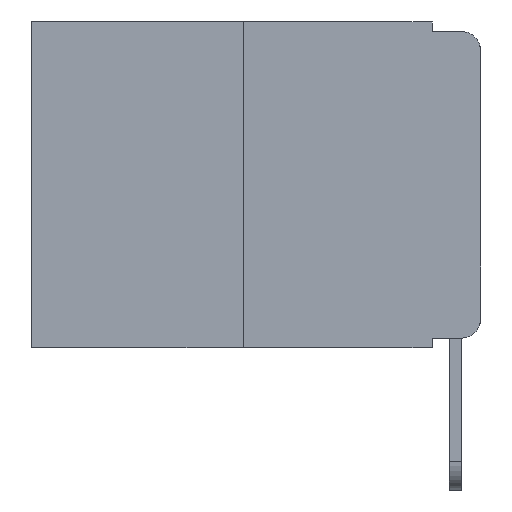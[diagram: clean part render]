
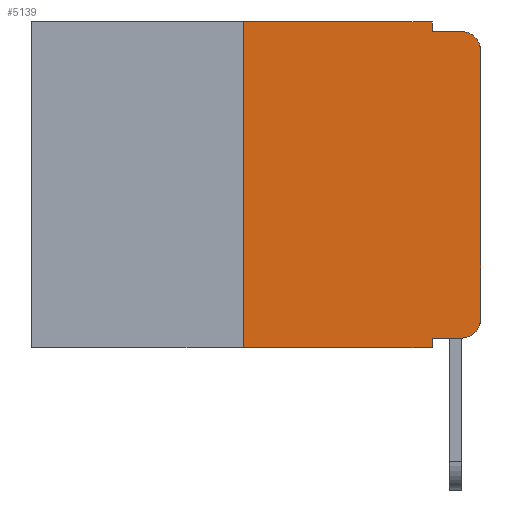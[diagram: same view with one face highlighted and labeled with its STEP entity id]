
A CAD part, left-side view. The second image highlights one B-rep face of the part: STEP entity #5139.
In plain terms, the highlighted planar face has unit normal (-1, 0, 0).
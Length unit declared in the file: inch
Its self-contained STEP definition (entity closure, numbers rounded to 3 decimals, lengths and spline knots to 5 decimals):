
#369 = DIRECTION ( 'NONE',  ( 0., 0., 1. ) ) ;
#731 = DIRECTION ( 'NONE',  ( 0., 0., 1. ) ) ;
#906 = AXIS2_PLACEMENT_3D ( 'NONE', #6692, #8714, #2921 ) ;
#1438 = VERTEX_POINT ( 'NONE', #13425 ) ;
#1613 = ORIENTED_EDGE ( 'NONE', *, *, #2578, .F. ) ;
#1664 = VERTEX_POINT ( 'NONE', #3669 ) ;
#1966 = CARTESIAN_POINT ( 'NONE',  ( 0., 0.051, 0. ) ) ;
#2036 = DIRECTION ( 'NONE',  ( 0., 0., -1. ) ) ;
#2057 = VERTEX_POINT ( 'NONE', #5916 ) ;
#2065 = EDGE_CURVE ( 'NONE', #4809, #1664, #3626, .T. ) ;
#2370 = EDGE_CURVE ( 'NONE', #10915, #11073, #7590, .T. ) ;
#2481 = CARTESIAN_POINT ( 'NONE',  ( 0., 0., -0.313 ) ) ;
#2497 = DIRECTION ( 'NONE',  ( 0., 0., -1. ) ) ;
#2549 = EDGE_CURVE ( 'NONE', #7358, #14684, #6705, .T. ) ;
#2551 = EDGE_CURVE ( 'NONE', #14684, #2057, #7060, .T. ) ;
#2554 = EDGE_CURVE ( 'NONE', #13820, #2057, #12006, .T. ) ;
#2575 = EDGE_CURVE ( 'NONE', #1664, #13820, #14382, .T. ) ;
#2578 = EDGE_CURVE ( 'NONE', #10915, #4809, #11686, .T. ) ;
#2579 = EDGE_CURVE ( 'NONE', #4024, #11073, #8967, .T. ) ;
#2598 = EDGE_CURVE ( 'NONE', #4024, #1438, #2799, .T. ) ;
#2606 = EDGE_CURVE ( 'NONE', #1438, #7358, #8618, .T. ) ;
#2672 = DIRECTION ( 'NONE',  ( -1., 0., 0. ) ) ;
#2799 = LINE ( 'NONE', #4948, #10291 ) ;
#2921 = DIRECTION ( 'NONE',  ( 0., 0., -1. ) ) ;
#3480 = DIRECTION ( 'NONE',  ( 0., -1., 0. ) ) ;
#3626 = LINE ( 'NONE', #5919, #9663 ) ;
#3650 = CARTESIAN_POINT ( 'NONE',  ( 0., 0.473, -0.343 ) ) ;
#3669 = CARTESIAN_POINT ( 'NONE',  ( 0., 0.051, 0. ) ) ;
#3837 = ORIENTED_EDGE ( 'NONE', *, *, #2549, .T. ) ;
#3870 = CARTESIAN_POINT ( 'NONE',  ( 0., 0.25, 0. ) ) ;
#4024 = VERTEX_POINT ( 'NONE', #11948 ) ;
#4524 = CARTESIAN_POINT ( 'NONE',  ( 0., 0.051, -0.01 ) ) ;
#4770 = DIRECTION ( 'NONE',  ( 0., 0., -1. ) ) ;
#4809 = VERTEX_POINT ( 'NONE', #9548 ) ;
#4843 = FACE_OUTER_BOUND ( 'NONE', #11471, .T. ) ;
#4948 = CARTESIAN_POINT ( 'NONE',  ( 0., 0.051, -0.333 ) ) ;
#5139 = ADVANCED_FACE ( 'NONE', ( #4843 ), #12438, .F. ) ;
#5342 = ORIENTED_EDGE ( 'NONE', *, *, #2579, .F. ) ;
#5916 = CARTESIAN_POINT ( 'NONE',  ( 0., 0.02, -0.01 ) ) ;
#5919 = CARTESIAN_POINT ( 'NONE',  ( 0., 0.473, 0. ) ) ;
#5983 = VECTOR ( 'NONE', #731, 39.37008 ) ;
#6352 = VECTOR ( 'NONE', #11063, 39.37008 ) ;
#6511 = CARTESIAN_POINT ( 'NONE',  ( 0., 0.051, -0.343 ) ) ;
#6692 = CARTESIAN_POINT ( 'NONE',  ( 0., 0.473, 0. ) ) ;
#6705 = LINE ( 'NONE', #7236, #7400 ) ;
#6944 = ORIENTED_EDGE ( 'NONE', *, *, #2551, .T. ) ;
#7009 = DIRECTION ( 'NONE',  ( -1., 0., 0. ) ) ;
#7060 = CIRCLE ( 'NONE', #11048, 0.02 ) ;
#7236 = CARTESIAN_POINT ( 'NONE',  ( 0., 0., 0. ) ) ;
#7294 = ORIENTED_EDGE ( 'NONE', *, *, #2554, .F. ) ;
#7358 = VERTEX_POINT ( 'NONE', #2481 ) ;
#7400 = VECTOR ( 'NONE', #369, 39.37008 ) ;
#7590 = LINE ( 'NONE', #3650, #13443 ) ;
#8342 = ORIENTED_EDGE ( 'NONE', *, *, #2598, .T. ) ;
#8618 = CIRCLE ( 'NONE', #12401, 0.02 ) ;
#8687 = ORIENTED_EDGE ( 'NONE', *, *, #2606, .T. ) ;
#8714 = DIRECTION ( 'NONE',  ( 1., 0., 0. ) ) ;
#8851 = CARTESIAN_POINT ( 'NONE',  ( 0., 0.051, 0. ) ) ;
#8967 = LINE ( 'NONE', #1966, #14068 ) ;
#9309 = VECTOR ( 'NONE', #4770, 39.37008 ) ;
#9514 = CARTESIAN_POINT ( 'NONE',  ( 0., 0.25, -0.343 ) ) ;
#9548 = CARTESIAN_POINT ( 'NONE',  ( 0., 0.25, 0. ) ) ;
#9663 = VECTOR ( 'NONE', #13832, 39.37008 ) ;
#10291 = VECTOR ( 'NONE', #14452, 39.37008 ) ;
#10454 = ORIENTED_EDGE ( 'NONE', *, *, #2575, .F. ) ;
#10769 = ORIENTED_EDGE ( 'NONE', *, *, #2370, .T. ) ;
#10785 = DIRECTION ( 'NONE',  ( 0., 0., -1. ) ) ;
#10915 = VERTEX_POINT ( 'NONE', #9514 ) ;
#11015 = CARTESIAN_POINT ( 'NONE',  ( 0., 0.051, -0.01 ) ) ;
#11048 = AXIS2_PLACEMENT_3D ( 'NONE', #14656, #7009, #2497 ) ;
#11063 = DIRECTION ( 'NONE',  ( 0., -1., 0. ) ) ;
#11073 = VERTEX_POINT ( 'NONE', #6511 ) ;
#11471 = EDGE_LOOP ( 'NONE', ( #3837, #6944, #7294, #10454, #13171, #1613, #10769, #5342, #8342, #8687 ) ) ;
#11686 = LINE ( 'NONE', #3870, #5983 ) ;
#11948 = CARTESIAN_POINT ( 'NONE',  ( 0., 0.051, -0.333 ) ) ;
#12006 = LINE ( 'NONE', #11015, #6352 ) ;
#12401 = AXIS2_PLACEMENT_3D ( 'NONE', #12804, #2672, #10785 ) ;
#12438 = PLANE ( 'NONE',  #906 ) ;
#12804 = CARTESIAN_POINT ( 'NONE',  ( 0., 0.02, -0.313 ) ) ;
#13171 = ORIENTED_EDGE ( 'NONE', *, *, #2065, .F. ) ;
#13425 = CARTESIAN_POINT ( 'NONE',  ( 0., 0.02, -0.333 ) ) ;
#13443 = VECTOR ( 'NONE', #3480, 39.37008 ) ;
#13820 = VERTEX_POINT ( 'NONE', #4524 ) ;
#13832 = DIRECTION ( 'NONE',  ( 0., -1., 0. ) ) ;
#14068 = VECTOR ( 'NONE', #2036, 39.37008 ) ;
#14382 = LINE ( 'NONE', #8851, #9309 ) ;
#14447 = CARTESIAN_POINT ( 'NONE',  ( 0., 0., -0.03 ) ) ;
#14452 = DIRECTION ( 'NONE',  ( 0., -1., 0. ) ) ;
#14656 = CARTESIAN_POINT ( 'NONE',  ( 0., 0.02, -0.03 ) ) ;
#14684 = VERTEX_POINT ( 'NONE', #14447 ) ;
